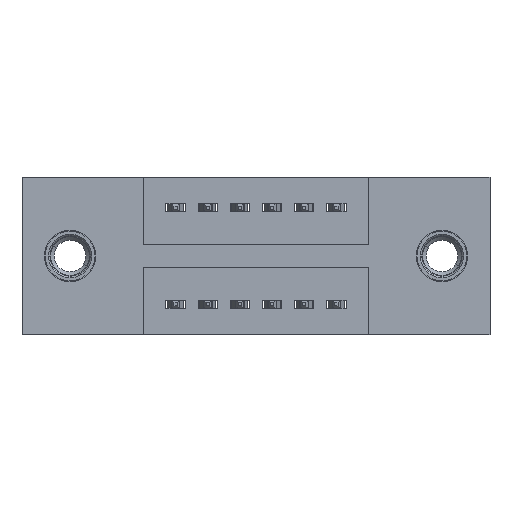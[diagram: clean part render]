
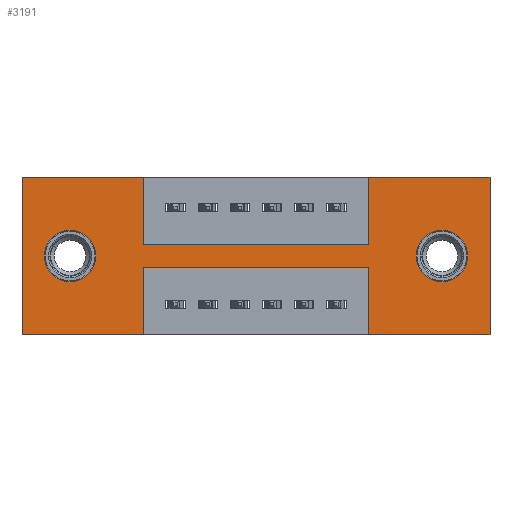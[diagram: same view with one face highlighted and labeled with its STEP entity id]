
A CAD part, front view. The second image highlights one B-rep face of the part: STEP entity #3191.
In plain terms, the highlighted planar face has unit normal (0, -1, 0).
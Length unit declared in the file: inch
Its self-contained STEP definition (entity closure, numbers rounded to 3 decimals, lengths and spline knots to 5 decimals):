
#60 = CARTESIAN_POINT ( 'NONE',  ( 0.3775, 0., -0.49 ) ) ;
#65 = VERTEX_POINT ( 'NONE', #6359 ) ;
#88 = VECTOR ( 'NONE', #2520, 39.37008 ) ;
#126 = CARTESIAN_POINT ( 'NONE',  ( 0.1495, 0., -0.325 ) ) ;
#147 = LINE ( 'NONE', #2782, #8731 ) ;
#179 = EDGE_CURVE ( 'NONE', #2877, #5684, #8236, .T. ) ;
#188 = VERTEX_POINT ( 'NONE', #6694 ) ;
#202 = EDGE_CURVE ( 'NONE', #569, #2322, #7179, .T. ) ;
#263 = CARTESIAN_POINT ( 'NONE',  ( 0., 0., 0. ) ) ;
#502 = ORIENTED_EDGE ( 'NONE', *, *, #2284, .F. ) ;
#562 = LINE ( 'NONE', #2972, #5029 ) ;
#569 = VERTEX_POINT ( 'NONE', #2143 ) ;
#716 = LINE ( 'NONE', #9160, #1978 ) ;
#722 = VERTEX_POINT ( 'NONE', #126 ) ;
#762 = ORIENTED_EDGE ( 'NONE', *, *, #8003, .T. ) ;
#782 = ORIENTED_EDGE ( 'NONE', *, *, #3646, .T. ) ;
#810 = CARTESIAN_POINT ( 'NONE',  ( 0.3775, 0., -0.28 ) ) ;
#848 = AXIS2_PLACEMENT_3D ( 'NONE', #2814, #8081, #3576 ) ;
#891 = CARTESIAN_POINT ( 'NONE',  ( 0., 0., -0.49 ) ) ;
#1061 = LINE ( 'NONE', #1394, #8709 ) ;
#1087 = CARTESIAN_POINT ( 'NONE',  ( 1.3055, 0., -0.325 ) ) ;
#1099 = VERTEX_POINT ( 'NONE', #1527 ) ;
#1126 = FACE_BOUND ( 'NONE', #2752, .T. ) ;
#1168 = ORIENTED_EDGE ( 'NONE', *, *, #5804, .F. ) ;
#1337 = CARTESIAN_POINT ( 'NONE',  ( 0., 0., -0.49 ) ) ;
#1341 = DIRECTION ( 'NONE',  ( 0., 0., 1. ) ) ;
#1350 = ORIENTED_EDGE ( 'NONE', *, *, #9358, .F. ) ;
#1365 = ORIENTED_EDGE ( 'NONE', *, *, #202, .F. ) ;
#1394 = CARTESIAN_POINT ( 'NONE',  ( 0.3775, 0., -0.28 ) ) ;
#1417 = CARTESIAN_POINT ( 'NONE',  ( 1.3055, 0., -0.245 ) ) ;
#1527 = CARTESIAN_POINT ( 'NONE',  ( 1.0775, 0., -0.49 ) ) ;
#1835 = DIRECTION ( 'NONE',  ( 0., 0., 1. ) ) ;
#1978 = VECTOR ( 'NONE', #3954, 39.37008 ) ;
#2027 = EDGE_CURVE ( 'NONE', #8046, #8686, #4780, .T. ) ;
#2143 = CARTESIAN_POINT ( 'NONE',  ( 1.0775, 0., 0. ) ) ;
#2191 = LINE ( 'NONE', #810, #5267 ) ;
#2251 = ORIENTED_EDGE ( 'NONE', *, *, #9638, .F. ) ;
#2284 = EDGE_CURVE ( 'NONE', #188, #5222, #2191, .T. ) ;
#2319 = CARTESIAN_POINT ( 'NONE',  ( 0.1495, 0., -0.245 ) ) ;
#2322 = VERTEX_POINT ( 'NONE', #5968 ) ;
#2360 = VERTEX_POINT ( 'NONE', #9123 ) ;
#2474 = AXIS2_PLACEMENT_3D ( 'NONE', #5875, #9012, #3742 ) ;
#2520 = DIRECTION ( 'NONE',  ( 1., 0., 0. ) ) ;
#2752 = EDGE_LOOP ( 'NONE', ( #5963, #782 ) ) ;
#2782 = CARTESIAN_POINT ( 'NONE',  ( 1.455, 0., 0. ) ) ;
#2814 = CARTESIAN_POINT ( 'NONE',  ( 0.1495, 0., -0.245 ) ) ;
#2870 = CARTESIAN_POINT ( 'NONE',  ( 0.1495, 0., -0.165 ) ) ;
#2877 = VERTEX_POINT ( 'NONE', #4902 ) ;
#2883 = FACE_OUTER_BOUND ( 'NONE', #4871, .T. ) ;
#2972 = CARTESIAN_POINT ( 'NONE',  ( 0.3775, 0., -0.21 ) ) ;
#3110 = FACE_BOUND ( 'NONE', #7443, .T. ) ;
#3191 = ADVANCED_FACE ( 'NONE', ( #1126, #3110, #2883 ), #6709, .T. ) ;
#3576 = DIRECTION ( 'NONE',  ( 0., 0., 1. ) ) ;
#3646 = EDGE_CURVE ( 'NONE', #5684, #2877, #6190, .T. ) ;
#3742 = DIRECTION ( 'NONE',  ( 0., 0., -1. ) ) ;
#3954 = DIRECTION ( 'NONE',  ( 1., 0., 0. ) ) ;
#3972 = CARTESIAN_POINT ( 'NONE',  ( 0., 0., 0. ) ) ;
#4297 = DIRECTION ( 'NONE',  ( -1., 0., 0. ) ) ;
#4331 = DIRECTION ( 'NONE',  ( 0., 0., -1. ) ) ;
#4536 = CARTESIAN_POINT ( 'NONE',  ( 0., 0., 0. ) ) ;
#4780 = LINE ( 'NONE', #263, #88 ) ;
#4871 = EDGE_LOOP ( 'NONE', ( #2251, #9346, #1350, #9096, #5307, #1168, #502, #7057, #7134, #7998, #6576, #1365 ) ) ;
#4902 = CARTESIAN_POINT ( 'NONE',  ( 1.3055, 0., -0.165 ) ) ;
#5024 = VECTOR ( 'NONE', #8273, 39.37008 ) ;
#5029 = VECTOR ( 'NONE', #5984, 39.37008 ) ;
#5112 = AXIS2_PLACEMENT_3D ( 'NONE', #2319, #7527, #7593 ) ;
#5124 = DIRECTION ( 'NONE',  ( 0., -1., 0. ) ) ;
#5143 = VECTOR ( 'NONE', #1835, 39.37008 ) ;
#5204 = EDGE_CURVE ( 'NONE', #2322, #8383, #147, .T. ) ;
#5222 = VERTEX_POINT ( 'NONE', #60 ) ;
#5267 = VECTOR ( 'NONE', #9051, 39.37008 ) ;
#5270 = DIRECTION ( 'NONE',  ( 0., 1., 0. ) ) ;
#5307 = ORIENTED_EDGE ( 'NONE', *, *, #9256, .F. ) ;
#5654 = LINE ( 'NONE', #891, #9312 ) ;
#5684 = VERTEX_POINT ( 'NONE', #1087 ) ;
#5772 = EDGE_CURVE ( 'NONE', #8383, #1099, #5654, .T. ) ;
#5804 = EDGE_CURVE ( 'NONE', #5222, #2360, #9077, .T. ) ;
#5812 = ORIENTED_EDGE ( 'NONE', *, *, #8382, .T. ) ;
#5875 = CARTESIAN_POINT ( 'NONE',  ( 1.3055, 0., -0.245 ) ) ;
#5963 = ORIENTED_EDGE ( 'NONE', *, *, #179, .T. ) ;
#5968 = CARTESIAN_POINT ( 'NONE',  ( 1.455, 0., 0. ) ) ;
#5973 = LINE ( 'NONE', #8993, #5024 ) ;
#5984 = DIRECTION ( 'NONE',  ( 0., 0., -1. ) ) ;
#6063 = DIRECTION ( 'NONE',  ( 1., 0., 0. ) ) ;
#6137 = CARTESIAN_POINT ( 'NONE',  ( 0.3775, 0., 0. ) ) ;
#6190 = CIRCLE ( 'NONE', #2474, 0.08 ) ;
#6353 = VECTOR ( 'NONE', #6063, 39.37008 ) ;
#6359 = CARTESIAN_POINT ( 'NONE',  ( 1.0775, 0., -0.21 ) ) ;
#6475 = CARTESIAN_POINT ( 'NONE',  ( 0., 0., -0.49 ) ) ;
#6576 = ORIENTED_EDGE ( 'NONE', *, *, #5204, .F. ) ;
#6694 = CARTESIAN_POINT ( 'NONE',  ( 0.3775, 0., -0.28 ) ) ;
#6709 = PLANE ( 'NONE',  #9040 ) ;
#6824 = DIRECTION ( 'NONE',  ( 0., 0., -1. ) ) ;
#6884 = EDGE_CURVE ( 'NONE', #7590, #65, #716, .T. ) ;
#6932 = VECTOR ( 'NONE', #1341, 39.37008 ) ;
#7057 = ORIENTED_EDGE ( 'NONE', *, *, #7133, .F. ) ;
#7133 = EDGE_CURVE ( 'NONE', #8670, #188, #1061, .T. ) ;
#7134 = ORIENTED_EDGE ( 'NONE', *, *, #8561, .F. ) ;
#7141 = VERTEX_POINT ( 'NONE', #2870 ) ;
#7179 = LINE ( 'NONE', #4536, #6353 ) ;
#7413 = DIRECTION ( 'NONE',  ( -1., 0., 0. ) ) ;
#7443 = EDGE_LOOP ( 'NONE', ( #5812, #762 ) ) ;
#7527 = DIRECTION ( 'NONE',  ( 0., 1., 0. ) ) ;
#7590 = VERTEX_POINT ( 'NONE', #7861 ) ;
#7593 = DIRECTION ( 'NONE',  ( 0., 0., 1. ) ) ;
#7612 = CARTESIAN_POINT ( 'NONE',  ( 1.0775, 0., -0.28 ) ) ;
#7733 = LINE ( 'NONE', #8085, #6932 ) ;
#7841 = LINE ( 'NONE', #9291, #5143 ) ;
#7852 = CIRCLE ( 'NONE', #848, 0.08 ) ;
#7861 = CARTESIAN_POINT ( 'NONE',  ( 0.3775, 0., -0.21 ) ) ;
#7998 = ORIENTED_EDGE ( 'NONE', *, *, #5772, .F. ) ;
#8003 = EDGE_CURVE ( 'NONE', #722, #7141, #9387, .T. ) ;
#8046 = VERTEX_POINT ( 'NONE', #3972 ) ;
#8048 = CARTESIAN_POINT ( 'NONE',  ( 1.455, 0., -0.49 ) ) ;
#8081 = DIRECTION ( 'NONE',  ( 0., 1., 0. ) ) ;
#8085 = CARTESIAN_POINT ( 'NONE',  ( 0., 0., 0. ) ) ;
#8236 = CIRCLE ( 'NONE', #8776, 0.08 ) ;
#8273 = DIRECTION ( 'NONE',  ( 0., 0., 1. ) ) ;
#8382 = EDGE_CURVE ( 'NONE', #7141, #722, #7852, .T. ) ;
#8383 = VERTEX_POINT ( 'NONE', #8048 ) ;
#8418 = DIRECTION ( 'NONE',  ( -1., 0., 0. ) ) ;
#8561 = EDGE_CURVE ( 'NONE', #1099, #8670, #5973, .T. ) ;
#8670 = VERTEX_POINT ( 'NONE', #7612 ) ;
#8686 = VERTEX_POINT ( 'NONE', #6137 ) ;
#8709 = VECTOR ( 'NONE', #7413, 39.37008 ) ;
#8731 = VECTOR ( 'NONE', #8960, 39.37008 ) ;
#8776 = AXIS2_PLACEMENT_3D ( 'NONE', #1417, #5270, #6824 ) ;
#8950 = VECTOR ( 'NONE', #4297, 39.37008 ) ;
#8960 = DIRECTION ( 'NONE',  ( 0., 0., -1. ) ) ;
#8993 = CARTESIAN_POINT ( 'NONE',  ( 1.0775, 0., -0.28 ) ) ;
#9012 = DIRECTION ( 'NONE',  ( 0., 1., 0. ) ) ;
#9040 = AXIS2_PLACEMENT_3D ( 'NONE', #1337, #5124, #4331 ) ;
#9051 = DIRECTION ( 'NONE',  ( 0., 0., -1. ) ) ;
#9077 = LINE ( 'NONE', #6475, #8950 ) ;
#9096 = ORIENTED_EDGE ( 'NONE', *, *, #2027, .F. ) ;
#9123 = CARTESIAN_POINT ( 'NONE',  ( 0., 0., -0.49 ) ) ;
#9160 = CARTESIAN_POINT ( 'NONE',  ( 0.3775, 0., -0.21 ) ) ;
#9256 = EDGE_CURVE ( 'NONE', #2360, #8046, #7733, .T. ) ;
#9291 = CARTESIAN_POINT ( 'NONE',  ( 1.0775, 0., -0.21 ) ) ;
#9312 = VECTOR ( 'NONE', #8418, 39.37008 ) ;
#9346 = ORIENTED_EDGE ( 'NONE', *, *, #6884, .F. ) ;
#9358 = EDGE_CURVE ( 'NONE', #8686, #7590, #562, .T. ) ;
#9387 = CIRCLE ( 'NONE', #5112, 0.08 ) ;
#9638 = EDGE_CURVE ( 'NONE', #65, #569, #7841, .T. ) ;
